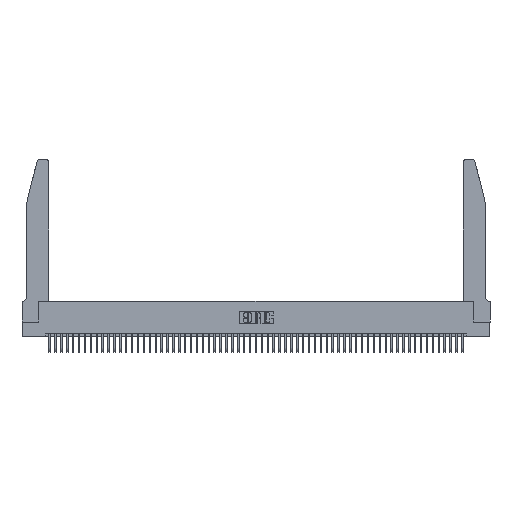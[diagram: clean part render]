
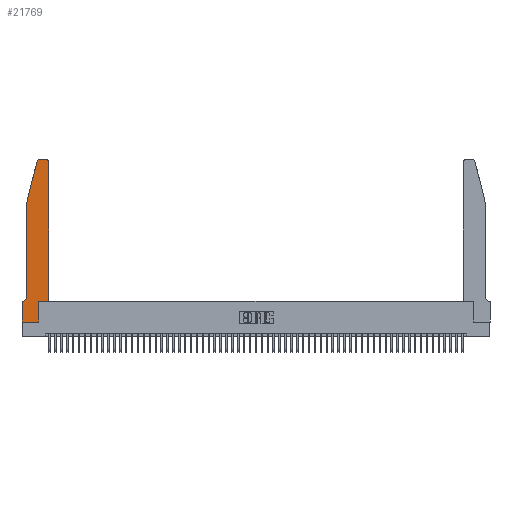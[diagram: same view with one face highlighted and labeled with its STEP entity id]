
A CAD part, top view. The second image highlights one B-rep face of the part: STEP entity #21769.
In plain terms, the highlighted planar face has unit normal (0, 0, 1).
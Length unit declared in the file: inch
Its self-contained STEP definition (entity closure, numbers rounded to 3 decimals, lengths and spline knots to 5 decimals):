
#512 = CARTESIAN_POINT ( 'NONE',  ( 0.0755, 2., 0.37 ) ) ;
#533 = EDGE_CURVE ( 'NONE', #52177, #49933, #14885, .T. ) ;
#689 = CARTESIAN_POINT ( 'NONE',  ( 0.0755, 0.42, 0.37 ) ) ;
#762 = ORIENTED_EDGE ( 'NONE', *, *, #51603, .T. ) ;
#1448 = CARTESIAN_POINT ( 'NONE',  ( 0.4505, 0.35, 0.37 ) ) ;
#2710 = ORIENTED_EDGE ( 'NONE', *, *, #4791, .T. ) ;
#3694 = VERTEX_POINT ( 'NONE', #12842 ) ;
#4791 = EDGE_CURVE ( 'NONE', #5745, #20338, #36788, .T. ) ;
#5411 = CIRCLE ( 'NONE', #17183, 0.03 ) ;
#5622 = LINE ( 'NONE', #17248, #48927 ) ;
#5671 = ORIENTED_EDGE ( 'NONE', *, *, #32210, .T. ) ;
#5709 = VECTOR ( 'NONE', #52754, 39.37008 ) ;
#5745 = VERTEX_POINT ( 'NONE', #53227 ) ;
#6139 = CARTESIAN_POINT ( 'NONE',  ( 0., 0., 0.37 ) ) ;
#6552 = CARTESIAN_POINT ( 'NONE',  ( 0.0755, 2., 0.37 ) ) ;
#6711 = EDGE_CURVE ( 'NONE', #20338, #52177, #19526, .T. ) ;
#7051 = DIRECTION ( 'NONE',  ( 0., 0., -1. ) ) ;
#8399 = CARTESIAN_POINT ( 'NONE',  ( 0.0755, 2., 0.37 ) ) ;
#9333 = CARTESIAN_POINT ( 'NONE',  ( 0.284, 2.72, 0.37 ) ) ;
#10215 = CARTESIAN_POINT ( 'NONE',  ( 0.2605, 2.75, 0.37 ) ) ;
#10542 = LINE ( 'NONE', #46922, #20423 ) ;
#10662 = ORIENTED_EDGE ( 'NONE', *, *, #33443, .T. ) ;
#12059 = ORIENTED_EDGE ( 'NONE', *, *, #14020, .T. ) ;
#12842 = CARTESIAN_POINT ( 'NONE',  ( 0.2865, 0.35, 0.37 ) ) ;
#13244 = DIRECTION ( 'NONE',  ( 0., -1., 0. ) ) ;
#13587 = DIRECTION ( 'NONE',  ( 1., 0., 0. ) ) ;
#13915 = AXIS2_PLACEMENT_3D ( 'NONE', #18257, #47551, #22484 ) ;
#14020 = EDGE_CURVE ( 'NONE', #20208, #39432, #36708, .T. ) ;
#14885 = LINE ( 'NONE', #512, #24712 ) ;
#16439 = EDGE_CURVE ( 'NONE', #19433, #3694, #5622, .T. ) ;
#16683 = VECTOR ( 'NONE', #41434, 39.37008 ) ;
#17183 = AXIS2_PLACEMENT_3D ( 'NONE', #20502, #49765, #24702 ) ;
#17248 = CARTESIAN_POINT ( 'NONE',  ( 0.2865, 0.35, 0.37 ) ) ;
#17421 = DIRECTION ( 'NONE',  ( 0., 1., 0. ) ) ;
#17642 = DIRECTION ( 'NONE',  ( 0., 1., 0. ) ) ;
#18024 = DIRECTION ( 'NONE',  ( 0., -1., 0. ) ) ;
#18257 = CARTESIAN_POINT ( 'NONE',  ( 0., 0.35, 0.37 ) ) ;
#18672 = DIRECTION ( 'NONE',  ( -1., 0., 0. ) ) ;
#19225 = LINE ( 'NONE', #10215, #40209 ) ;
#19433 = VERTEX_POINT ( 'NONE', #44583 ) ;
#19526 = LINE ( 'NONE', #6552, #5709 ) ;
#19785 = ORIENTED_EDGE ( 'NONE', *, *, #37061, .T. ) ;
#20205 = ORIENTED_EDGE ( 'NONE', *, *, #53455, .T. ) ;
#20208 = VERTEX_POINT ( 'NONE', #28383 ) ;
#20338 = VERTEX_POINT ( 'NONE', #37574 ) ;
#20423 = VECTOR ( 'NONE', #17642, 39.37008 ) ;
#20502 = CARTESIAN_POINT ( 'NONE',  ( 0.4205, 2.72, 0.37 ) ) ;
#20800 = DIRECTION ( 'NONE',  ( -1., 0., 0. ) ) ;
#20809 = CARTESIAN_POINT ( 'NONE',  ( 0.4505, 2.72, 0.37 ) ) ;
#21769 = ADVANCED_FACE ( 'NONE', ( #50325 ), #43358, .T. ) ;
#22337 = VERTEX_POINT ( 'NONE', #1448 ) ;
#22484 = DIRECTION ( 'NONE',  ( 1., 0., 0. ) ) ;
#23122 = ORIENTED_EDGE ( 'NONE', *, *, #6711, .T. ) ;
#24448 = AXIS2_PLACEMENT_3D ( 'NONE', #9333, #38694, #13587 ) ;
#24702 = DIRECTION ( 'NONE',  ( 1., 0., 0. ) ) ;
#24712 = VECTOR ( 'NONE', #13244, 39.37008 ) ;
#25513 = VECTOR ( 'NONE', #18024, 39.37008 ) ;
#25655 = CARTESIAN_POINT ( 'NONE',  ( 0.0055, 0.35, 0.37 ) ) ;
#26260 = CARTESIAN_POINT ( 'NONE',  ( 0., 0., 0.37 ) ) ;
#26509 = EDGE_LOOP ( 'NONE', ( #19785, #2710, #23122, #49303, #51267, #762, #12059, #53336, #39755, #20205, #10662, #5671 ) ) ;
#27791 = CARTESIAN_POINT ( 'NONE',  ( 0.4205, 2.75, 0.37 ) ) ;
#28289 = VERTEX_POINT ( 'NONE', #25655 ) ;
#28383 = CARTESIAN_POINT ( 'NONE',  ( 0., 0.35, 0.37 ) ) ;
#29178 = CARTESIAN_POINT ( 'NONE',  ( 0.0755, 0.35, 0.37 ) ) ;
#29886 = LINE ( 'NONE', #29178, #41094 ) ;
#30243 = CARTESIAN_POINT ( 'NONE',  ( 0., 0., 0.37 ) ) ;
#31264 = EDGE_CURVE ( 'NONE', #39432, #19433, #40322, .T. ) ;
#32203 = CARTESIAN_POINT ( 'NONE',  ( 0.0055, 0.42, 0.37 ) ) ;
#32210 = EDGE_CURVE ( 'NONE', #46787, #43588, #5411, .T. ) ;
#33003 = CARTESIAN_POINT ( 'NONE',  ( 0.4505, 0.35, 0.37 ) ) ;
#33443 = EDGE_CURVE ( 'NONE', #22337, #46787, #10542, .T. ) ;
#36429 = DIRECTION ( 'NONE',  ( -1., 0., 0. ) ) ;
#36708 = LINE ( 'NONE', #26260, #25513 ) ;
#36788 = CIRCLE ( 'NONE', #24448, 0.03 ) ;
#37061 = EDGE_CURVE ( 'NONE', #43588, #5745, #19225, .T. ) ;
#37574 = CARTESIAN_POINT ( 'NONE',  ( 0.25487, 2.72718, 0.37 ) ) ;
#38694 = DIRECTION ( 'NONE',  ( 0., 0., 1. ) ) ;
#38997 = VECTOR ( 'NONE', #51117, 39.37008 ) ;
#39432 = VERTEX_POINT ( 'NONE', #6139 ) ;
#39588 = EDGE_CURVE ( 'NONE', #49933, #28289, #45882, .T. ) ;
#39755 = ORIENTED_EDGE ( 'NONE', *, *, #16439, .T. ) ;
#40209 = VECTOR ( 'NONE', #18672, 39.37008 ) ;
#40322 = LINE ( 'NONE', #30243, #38997 ) ;
#41094 = VECTOR ( 'NONE', #20800, 39.37008 ) ;
#41434 = DIRECTION ( 'NONE',  ( 1., 0., 0. ) ) ;
#41999 = AXIS2_PLACEMENT_3D ( 'NONE', #32203, #7051, #36429 ) ;
#43358 = PLANE ( 'NONE',  #13915 ) ;
#43588 = VERTEX_POINT ( 'NONE', #27791 ) ;
#44583 = CARTESIAN_POINT ( 'NONE',  ( 0.2865, 0., 0.37 ) ) ;
#45882 = CIRCLE ( 'NONE', #41999, 0.07 ) ;
#46787 = VERTEX_POINT ( 'NONE', #20809 ) ;
#46922 = CARTESIAN_POINT ( 'NONE',  ( 0.4505, 0.35, 0.37 ) ) ;
#47551 = DIRECTION ( 'NONE',  ( 0., 0., 1. ) ) ;
#48927 = VECTOR ( 'NONE', #17421, 39.37008 ) ;
#49303 = ORIENTED_EDGE ( 'NONE', *, *, #533, .T. ) ;
#49765 = DIRECTION ( 'NONE',  ( 0., 0., 1. ) ) ;
#49933 = VERTEX_POINT ( 'NONE', #689 ) ;
#50095 = LINE ( 'NONE', #33003, #16683 ) ;
#50325 = FACE_OUTER_BOUND ( 'NONE', #26509, .T. ) ;
#51117 = DIRECTION ( 'NONE',  ( 1., 0., 0. ) ) ;
#51267 = ORIENTED_EDGE ( 'NONE', *, *, #39588, .T. ) ;
#51603 = EDGE_CURVE ( 'NONE', #28289, #20208, #29886, .T. ) ;
#52177 = VERTEX_POINT ( 'NONE', #8399 ) ;
#52754 = DIRECTION ( 'NONE',  ( -0.239, -0.971, 0. ) ) ;
#53227 = CARTESIAN_POINT ( 'NONE',  ( 0.284, 2.75, 0.37 ) ) ;
#53336 = ORIENTED_EDGE ( 'NONE', *, *, #31264, .T. ) ;
#53455 = EDGE_CURVE ( 'NONE', #3694, #22337, #50095, .T. ) ;
